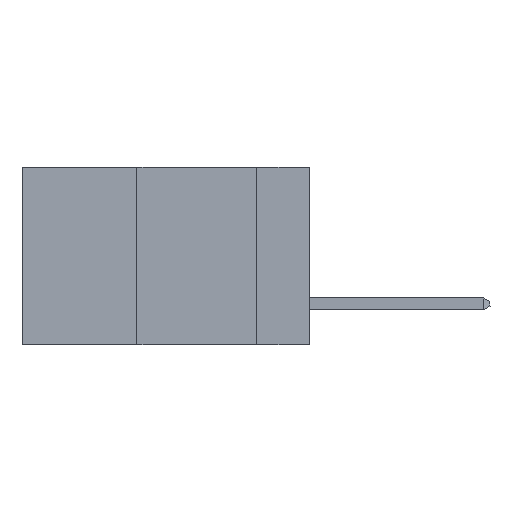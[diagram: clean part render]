
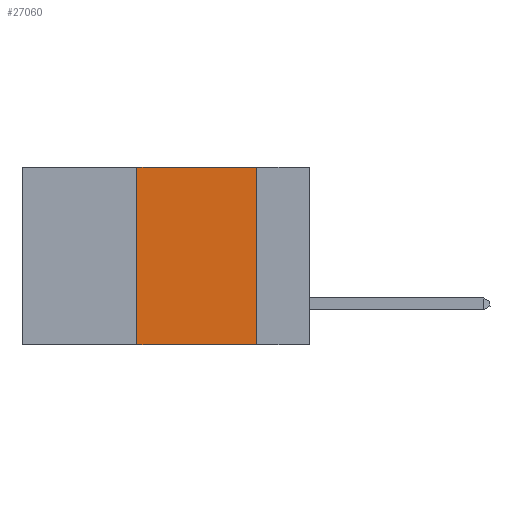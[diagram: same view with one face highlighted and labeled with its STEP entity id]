
A CAD part, left-side view. The second image highlights one B-rep face of the part: STEP entity #27060.
In plain terms, the highlighted planar face has unit normal (-1, 0, 0).
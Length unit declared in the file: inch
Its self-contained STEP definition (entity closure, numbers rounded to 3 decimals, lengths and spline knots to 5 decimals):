
#1073 = DIRECTION ( 'NONE',  ( 0., 0., -1. ) ) ;
#1603 = VERTEX_POINT ( 'NONE', #7391 ) ;
#1992 = VECTOR ( 'NONE', #17069, 39.37008 ) ;
#2735 = PLANE ( 'NONE',  #12774 ) ;
#2809 = ORIENTED_EDGE ( 'NONE', *, *, #24134, .F. ) ;
#3151 = LINE ( 'NONE', #26986, #25464 ) ;
#4554 = LINE ( 'NONE', #22754, #16108 ) ;
#4623 = CARTESIAN_POINT ( 'NONE',  ( 0., 0.36, -0.37 ) ) ;
#5358 = CARTESIAN_POINT ( 'NONE',  ( 0., 0.36, 0. ) ) ;
#5430 = VERTEX_POINT ( 'NONE', #7125 ) ;
#6457 = DIRECTION ( 'NONE',  ( 0., 0., 1. ) ) ;
#7125 = CARTESIAN_POINT ( 'NONE',  ( 0., 0.11, 0. ) ) ;
#7163 = DIRECTION ( 'NONE',  ( 1., 0., 0. ) ) ;
#7391 = CARTESIAN_POINT ( 'NONE',  ( 0., 0.11, -0.37 ) ) ;
#9096 = VERTEX_POINT ( 'NONE', #5358 ) ;
#9661 = EDGE_LOOP ( 'NONE', ( #2809, #26116, #13727, #22842 ) ) ;
#11247 = LINE ( 'NONE', #17258, #17711 ) ;
#12774 = AXIS2_PLACEMENT_3D ( 'NONE', #26347, #7163, #22275 ) ;
#12796 = EDGE_CURVE ( 'NONE', #9096, #5430, #14279, .T. ) ;
#13727 = ORIENTED_EDGE ( 'NONE', *, *, #16966, .F. ) ;
#14279 = LINE ( 'NONE', #27727, #1992 ) ;
#15494 = EDGE_CURVE ( 'NONE', #21261, #1603, #4554, .T. ) ;
#16108 = VECTOR ( 'NONE', #16361, 39.37008 ) ;
#16361 = DIRECTION ( 'NONE',  ( 0., -1., 0. ) ) ;
#16860 = FACE_OUTER_BOUND ( 'NONE', #9661, .T. ) ;
#16966 = EDGE_CURVE ( 'NONE', #21261, #9096, #11247, .T. ) ;
#17069 = DIRECTION ( 'NONE',  ( 0., -1., 0. ) ) ;
#17258 = CARTESIAN_POINT ( 'NONE',  ( 0., 0.36, 0. ) ) ;
#17711 = VECTOR ( 'NONE', #6457, 39.37008 ) ;
#21261 = VERTEX_POINT ( 'NONE', #4623 ) ;
#22275 = DIRECTION ( 'NONE',  ( 0., 0., -1. ) ) ;
#22754 = CARTESIAN_POINT ( 'NONE',  ( 0., 0.6, -0.37 ) ) ;
#22842 = ORIENTED_EDGE ( 'NONE', *, *, #15494, .T. ) ;
#24134 = EDGE_CURVE ( 'NONE', #5430, #1603, #3151, .T. ) ;
#25464 = VECTOR ( 'NONE', #1073, 39.37008 ) ;
#26116 = ORIENTED_EDGE ( 'NONE', *, *, #12796, .F. ) ;
#26347 = CARTESIAN_POINT ( 'NONE',  ( 0., 0.6, 0. ) ) ;
#26986 = CARTESIAN_POINT ( 'NONE',  ( 0., 0.11, 0. ) ) ;
#27060 = ADVANCED_FACE ( 'NONE', ( #16860 ), #2735, .F. ) ;
#27727 = CARTESIAN_POINT ( 'NONE',  ( 0., 0.6, 0. ) ) ;
